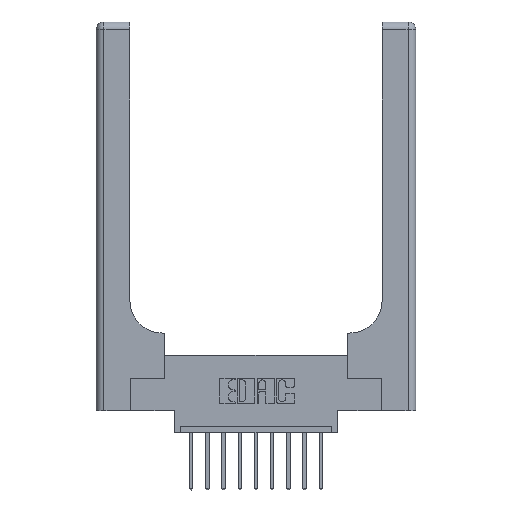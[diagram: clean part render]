
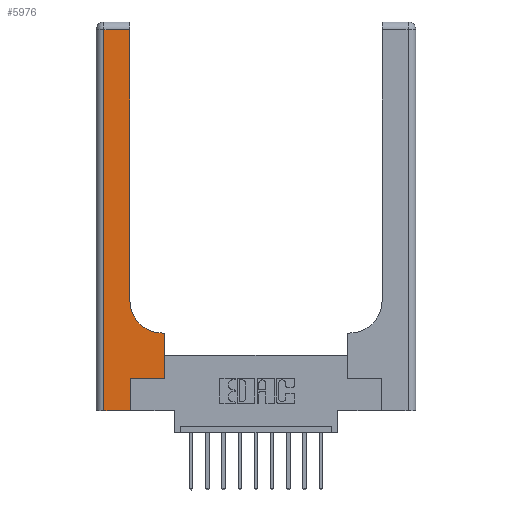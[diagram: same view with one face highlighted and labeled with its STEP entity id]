
A CAD part, top view. The second image highlights one B-rep face of the part: STEP entity #5976.
In plain terms, the highlighted planar face has unit normal (0, 0, 1).
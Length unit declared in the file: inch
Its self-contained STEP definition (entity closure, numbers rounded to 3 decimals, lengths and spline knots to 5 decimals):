
#23 = EDGE_CURVE ( 'NONE', #6780, #12561, #14350, .T. ) ;
#53 = DIRECTION ( 'NONE',  ( 0., -1., 0. ) ) ;
#150 = ORIENTED_EDGE ( 'NONE', *, *, #11361, .T. ) ;
#379 = CARTESIAN_POINT ( 'NONE',  ( 0.265, 0., 0.37 ) ) ;
#780 = EDGE_CURVE ( 'NONE', #7220, #8831, #5941, .T. ) ;
#881 = ORIENTED_EDGE ( 'NONE', *, *, #780, .T. ) ;
#989 = VECTOR ( 'NONE', #10047, 39.37008 ) ;
#1056 = VERTEX_POINT ( 'NONE', #14224 ) ;
#1794 = VECTOR ( 'NONE', #9844, 39.37008 ) ;
#1802 = EDGE_CURVE ( 'NONE', #7722, #7220, #7580, .T. ) ;
#2513 = CARTESIAN_POINT ( 'NONE',  ( 0.265, 0., 0.37 ) ) ;
#2767 = CARTESIAN_POINT ( 'NONE',  ( 0.528, 0.6, 0.37 ) ) ;
#3002 = EDGE_CURVE ( 'NONE', #9362, #7722, #8294, .T. ) ;
#3049 = VERTEX_POINT ( 'NONE', #4235 ) ;
#3364 = CARTESIAN_POINT ( 'NONE',  ( 0.06, 2.94, 0.37 ) ) ;
#3389 = PLANE ( 'NONE',  #4820 ) ;
#3408 = CARTESIAN_POINT ( 'NONE',  ( 0.26, 0.6, 0.37 ) ) ;
#3582 = ORIENTED_EDGE ( 'NONE', *, *, #5938, .T. ) ;
#3886 = VECTOR ( 'NONE', #11770, 39.37008 ) ;
#4235 = CARTESIAN_POINT ( 'NONE',  ( 0.26, 0.85, 0.37 ) ) ;
#4340 = VERTEX_POINT ( 'NONE', #3364 ) ;
#4365 = VECTOR ( 'NONE', #14560, 39.37008 ) ;
#4734 = CARTESIAN_POINT ( 'NONE',  ( 0.51, 0.85, 0.37 ) ) ;
#4797 = CARTESIAN_POINT ( 'NONE',  ( 0.528, 0.25, 0.37 ) ) ;
#4820 = AXIS2_PLACEMENT_3D ( 'NONE', #15377, #9448, #11853 ) ;
#5457 = EDGE_CURVE ( 'NONE', #3049, #1056, #7661, .T. ) ;
#5481 = ORIENTED_EDGE ( 'NONE', *, *, #13740, .T. ) ;
#5545 = CARTESIAN_POINT ( 'NONE',  ( 0., 2.94, 0.37 ) ) ;
#5889 = DIRECTION ( 'NONE',  ( 1., 0., 0. ) ) ;
#5938 = EDGE_CURVE ( 'NONE', #4340, #6780, #7184, .T. ) ;
#5941 = LINE ( 'NONE', #3408, #3886 ) ;
#5976 = ADVANCED_FACE ( 'NONE', ( #8823 ), #3389, .F. ) ;
#6737 = CARTESIAN_POINT ( 'NONE',  ( 0.06, 0., 0.37 ) ) ;
#6780 = VERTEX_POINT ( 'NONE', #6737 ) ;
#6901 = CIRCLE ( 'NONE', #9188, 0.25 ) ;
#7161 = CARTESIAN_POINT ( 'NONE',  ( 0.06, 3., 0.37 ) ) ;
#7184 = LINE ( 'NONE', #7161, #14730 ) ;
#7220 = VERTEX_POINT ( 'NONE', #2767 ) ;
#7580 = LINE ( 'NONE', #4797, #11488 ) ;
#7661 = LINE ( 'NONE', #8479, #989 ) ;
#7722 = VERTEX_POINT ( 'NONE', #10663 ) ;
#7805 = VECTOR ( 'NONE', #12664, 39.37008 ) ;
#7861 = VECTOR ( 'NONE', #9146, 39.37008 ) ;
#8294 = LINE ( 'NONE', #13453, #4365 ) ;
#8479 = CARTESIAN_POINT ( 'NONE',  ( 0.26, 3., 0.37 ) ) ;
#8823 = FACE_OUTER_BOUND ( 'NONE', #14711, .T. ) ;
#8831 = VERTEX_POINT ( 'NONE', #12050 ) ;
#9146 = DIRECTION ( 'NONE',  ( -1., 0., 0. ) ) ;
#9188 = AXIS2_PLACEMENT_3D ( 'NONE', #4734, #9502, #5889 ) ;
#9362 = VERTEX_POINT ( 'NONE', #15343 ) ;
#9448 = DIRECTION ( 'NONE',  ( 0., 0., -1. ) ) ;
#9502 = DIRECTION ( 'NONE',  ( 0., 0., -1. ) ) ;
#9596 = DIRECTION ( 'NONE',  ( 0., 1., 0. ) ) ;
#9844 = DIRECTION ( 'NONE',  ( 0., 1., 0. ) ) ;
#10047 = DIRECTION ( 'NONE',  ( 0., 1., 0. ) ) ;
#10635 = ORIENTED_EDGE ( 'NONE', *, *, #1802, .T. ) ;
#10663 = CARTESIAN_POINT ( 'NONE',  ( 0.528, 0.25, 0.37 ) ) ;
#11361 = EDGE_CURVE ( 'NONE', #12561, #9362, #12749, .T. ) ;
#11488 = VECTOR ( 'NONE', #9596, 39.37008 ) ;
#11770 = DIRECTION ( 'NONE',  ( -1., 0., 0. ) ) ;
#11853 = DIRECTION ( 'NONE',  ( -1., 0., 0. ) ) ;
#11903 = ORIENTED_EDGE ( 'NONE', *, *, #23, .T. ) ;
#12031 = ORIENTED_EDGE ( 'NONE', *, *, #5457, .T. ) ;
#12050 = CARTESIAN_POINT ( 'NONE',  ( 0.51, 0.6, 0.37 ) ) ;
#12329 = ORIENTED_EDGE ( 'NONE', *, *, #3002, .T. ) ;
#12561 = VERTEX_POINT ( 'NONE', #2513 ) ;
#12612 = CARTESIAN_POINT ( 'NONE',  ( 0., 0., 0.37 ) ) ;
#12664 = DIRECTION ( 'NONE',  ( 1., 0., 0. ) ) ;
#12749 = LINE ( 'NONE', #379, #1794 ) ;
#12956 = EDGE_CURVE ( 'NONE', #1056, #4340, #14389, .T. ) ;
#13453 = CARTESIAN_POINT ( 'NONE',  ( 0.265, 0.25, 0.37 ) ) ;
#13740 = EDGE_CURVE ( 'NONE', #8831, #3049, #6901, .T. ) ;
#14224 = CARTESIAN_POINT ( 'NONE',  ( 0.26, 2.94, 0.37 ) ) ;
#14350 = LINE ( 'NONE', #12612, #7805 ) ;
#14389 = LINE ( 'NONE', #5545, #7861 ) ;
#14560 = DIRECTION ( 'NONE',  ( 1., 0., 0. ) ) ;
#14697 = ORIENTED_EDGE ( 'NONE', *, *, #12956, .T. ) ;
#14711 = EDGE_LOOP ( 'NONE', ( #12031, #14697, #3582, #11903, #150, #12329, #10635, #881, #5481 ) ) ;
#14730 = VECTOR ( 'NONE', #53, 39.37008 ) ;
#15343 = CARTESIAN_POINT ( 'NONE',  ( 0.265, 0.25, 0.37 ) ) ;
#15377 = CARTESIAN_POINT ( 'NONE',  ( 0., 3., 0.37 ) ) ;
